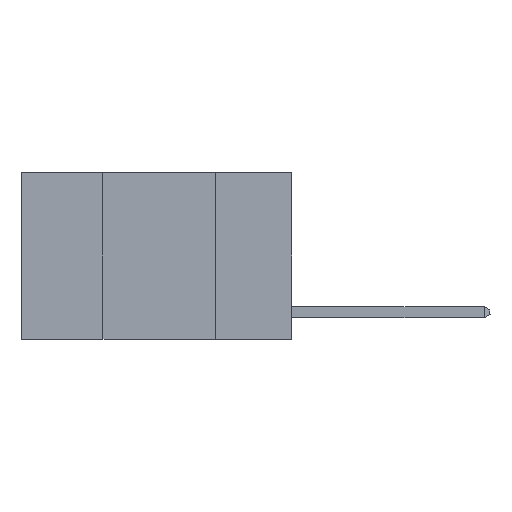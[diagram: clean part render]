
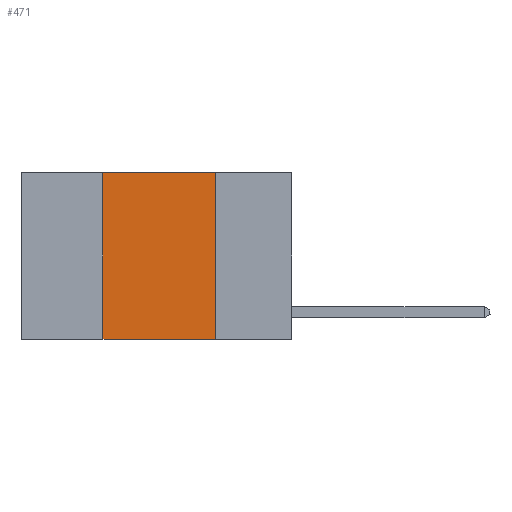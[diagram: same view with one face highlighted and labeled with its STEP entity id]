
A CAD part, left-side view. The second image highlights one B-rep face of the part: STEP entity #471.
In plain terms, the highlighted planar face has unit normal (-1, 0, 0).
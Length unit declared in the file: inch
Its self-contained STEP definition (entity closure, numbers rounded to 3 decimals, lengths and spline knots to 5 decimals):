
#334 = LINE ( 'NONE', #5361, #11084 ) ;
#471 = ADVANCED_FACE ( 'NONE', ( #9406 ), #12423, .F. ) ;
#574 = EDGE_LOOP ( 'NONE', ( #9640, #5420, #4102, #9243 ) ) ;
#1289 = EDGE_CURVE ( 'NONE', #3937, #4739, #10425, .T. ) ;
#1720 = DIRECTION ( 'NONE',  ( 0., -1., 0. ) ) ;
#2191 = VECTOR ( 'NONE', #6504, 39.37008 ) ;
#2383 = CARTESIAN_POINT ( 'NONE',  ( 0., 0.6, -0.37 ) ) ;
#2765 = AXIS2_PLACEMENT_3D ( 'NONE', #7633, #6615, #8518 ) ;
#3471 = LINE ( 'NONE', #2383, #2191 ) ;
#3937 = VERTEX_POINT ( 'NONE', #6367 ) ;
#4102 = ORIENTED_EDGE ( 'NONE', *, *, #10753, .F. ) ;
#4675 = VECTOR ( 'NONE', #1720, 39.37008 ) ;
#4739 = VERTEX_POINT ( 'NONE', #4981 ) ;
#4981 = CARTESIAN_POINT ( 'NONE',  ( 0., 0.17, 0. ) ) ;
#5159 = LINE ( 'NONE', #7153, #5664 ) ;
#5361 = CARTESIAN_POINT ( 'NONE',  ( 0., 0.17, 0. ) ) ;
#5420 = ORIENTED_EDGE ( 'NONE', *, *, #1289, .F. ) ;
#5664 = VECTOR ( 'NONE', #7213, 39.37008 ) ;
#6367 = CARTESIAN_POINT ( 'NONE',  ( 0., 0.42, 0. ) ) ;
#6400 = DIRECTION ( 'NONE',  ( 0., 0., -1. ) ) ;
#6504 = DIRECTION ( 'NONE',  ( 0., -1., 0. ) ) ;
#6615 = DIRECTION ( 'NONE',  ( 1., 0., 0. ) ) ;
#6648 = CARTESIAN_POINT ( 'NONE',  ( 0., 0.6, 0. ) ) ;
#7153 = CARTESIAN_POINT ( 'NONE',  ( 0., 0.42, 0. ) ) ;
#7164 = CARTESIAN_POINT ( 'NONE',  ( 0., 0.17, -0.37 ) ) ;
#7213 = DIRECTION ( 'NONE',  ( 0., 0., 1. ) ) ;
#7633 = CARTESIAN_POINT ( 'NONE',  ( 0., 0.6, 0. ) ) ;
#7707 = EDGE_CURVE ( 'NONE', #4739, #9105, #334, .T. ) ;
#8319 = CARTESIAN_POINT ( 'NONE',  ( 0., 0.42, -0.37 ) ) ;
#8518 = DIRECTION ( 'NONE',  ( 0., 0., -1. ) ) ;
#9105 = VERTEX_POINT ( 'NONE', #7164 ) ;
#9243 = ORIENTED_EDGE ( 'NONE', *, *, #11589, .T. ) ;
#9406 = FACE_OUTER_BOUND ( 'NONE', #574, .T. ) ;
#9640 = ORIENTED_EDGE ( 'NONE', *, *, #7707, .F. ) ;
#10123 = VERTEX_POINT ( 'NONE', #8319 ) ;
#10425 = LINE ( 'NONE', #6648, #4675 ) ;
#10753 = EDGE_CURVE ( 'NONE', #10123, #3937, #5159, .T. ) ;
#11084 = VECTOR ( 'NONE', #6400, 39.37008 ) ;
#11589 = EDGE_CURVE ( 'NONE', #10123, #9105, #3471, .T. ) ;
#12423 = PLANE ( 'NONE',  #2765 ) ;
